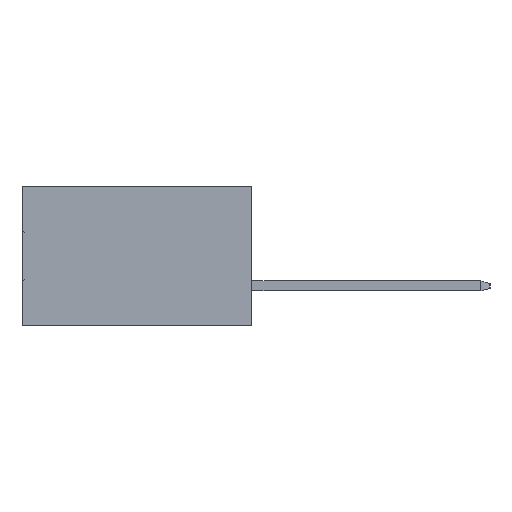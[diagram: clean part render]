
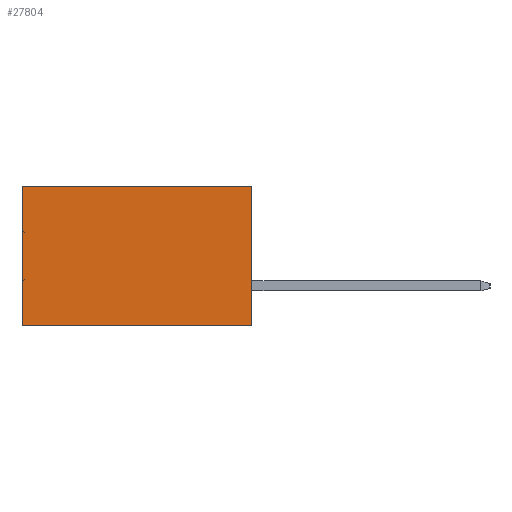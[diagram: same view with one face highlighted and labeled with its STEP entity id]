
A CAD part, left-side view. The second image highlights one B-rep face of the part: STEP entity #27804.
In plain terms, the highlighted planar face has unit normal (-1, 0, 0).
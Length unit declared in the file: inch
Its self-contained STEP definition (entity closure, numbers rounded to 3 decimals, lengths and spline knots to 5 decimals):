
#369 = EDGE_CURVE ( 'NONE', #15419, #2370, #13715, .T. ) ;
#1875 = ORIENTED_EDGE ( 'NONE', *, *, #20139, .T. ) ;
#2370 = VERTEX_POINT ( 'NONE', #21059 ) ;
#5299 = LINE ( 'NONE', #9087, #12865 ) ;
#6203 = VECTOR ( 'NONE', #17572, 39.37008 ) ;
#8636 = FACE_OUTER_BOUND ( 'NONE', #11217, .T. ) ;
#8965 = LINE ( 'NONE', #13344, #6203 ) ;
#9087 = CARTESIAN_POINT ( 'NONE',  ( 0.3205, 0., -0.437 ) ) ;
#9483 = VERTEX_POINT ( 'NONE', #11201 ) ;
#11201 = CARTESIAN_POINT ( 'NONE',  ( 0.3205, 0., 0. ) ) ;
#11217 = EDGE_LOOP ( 'NONE', ( #18207, #15017, #27690, #1875 ) ) ;
#11406 = LINE ( 'NONE', #14173, #17368 ) ;
#12510 = AXIS2_PLACEMENT_3D ( 'NONE', #28767, #15619, #24393 ) ;
#12865 = VECTOR ( 'NONE', #13901, 39.37008 ) ;
#13029 = PLANE ( 'NONE',  #12510 ) ;
#13344 = CARTESIAN_POINT ( 'NONE',  ( 0.3205, 0., -0.437 ) ) ;
#13715 = LINE ( 'NONE', #22604, #14392 ) ;
#13901 = DIRECTION ( 'NONE',  ( 0., 1., 0. ) ) ;
#14173 = CARTESIAN_POINT ( 'NONE',  ( 0.3205, 0., 0. ) ) ;
#14392 = VECTOR ( 'NONE', #20430, 39.37008 ) ;
#15017 = ORIENTED_EDGE ( 'NONE', *, *, #24831, .F. ) ;
#15419 = VERTEX_POINT ( 'NONE', #21346 ) ;
#15619 = DIRECTION ( 'NONE',  ( 1., 0., 0. ) ) ;
#17368 = VECTOR ( 'NONE', #20311, 39.37008 ) ;
#17572 = DIRECTION ( 'NONE',  ( 0., 0., -1. ) ) ;
#18207 = ORIENTED_EDGE ( 'NONE', *, *, #369, .T. ) ;
#19682 = EDGE_CURVE ( 'NONE', #9483, #23352, #8965, .T. ) ;
#19904 = CARTESIAN_POINT ( 'NONE',  ( 0.3205, 0., -0.437 ) ) ;
#20139 = EDGE_CURVE ( 'NONE', #9483, #15419, #11406, .T. ) ;
#20311 = DIRECTION ( 'NONE',  ( 0., 1., 0. ) ) ;
#20430 = DIRECTION ( 'NONE',  ( 0., 0., -1. ) ) ;
#21059 = CARTESIAN_POINT ( 'NONE',  ( 0.3205, 0.72, -0.437 ) ) ;
#21346 = CARTESIAN_POINT ( 'NONE',  ( 0.3205, 0.72, 0. ) ) ;
#22604 = CARTESIAN_POINT ( 'NONE',  ( 0.3205, 0.72, -0.437 ) ) ;
#23352 = VERTEX_POINT ( 'NONE', #19904 ) ;
#24393 = DIRECTION ( 'NONE',  ( 0., 0., -1. ) ) ;
#24831 = EDGE_CURVE ( 'NONE', #23352, #2370, #5299, .T. ) ;
#27690 = ORIENTED_EDGE ( 'NONE', *, *, #19682, .F. ) ;
#27804 = ADVANCED_FACE ( 'NONE', ( #8636 ), #13029, .F. ) ;
#28767 = CARTESIAN_POINT ( 'NONE',  ( 0.3205, 0., -0.437 ) ) ;
